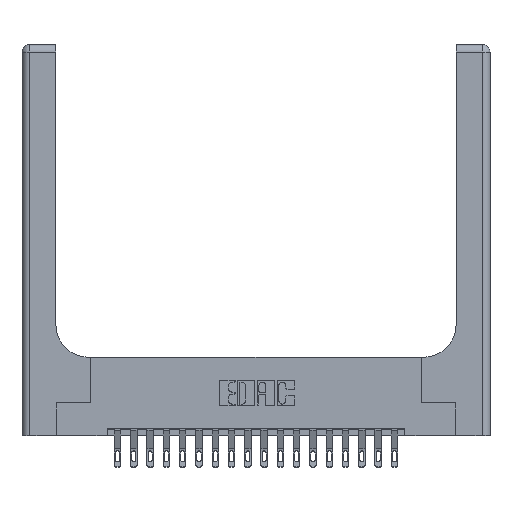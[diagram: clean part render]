
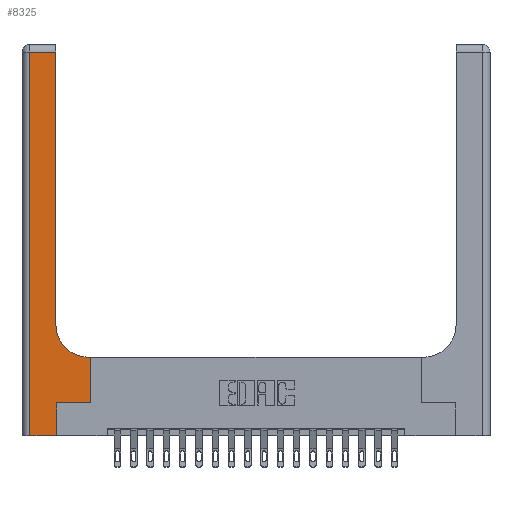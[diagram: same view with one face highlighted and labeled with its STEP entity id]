
A CAD part, top view. The second image highlights one B-rep face of the part: STEP entity #8325.
In plain terms, the highlighted planar face has unit normal (0, 0, 1).
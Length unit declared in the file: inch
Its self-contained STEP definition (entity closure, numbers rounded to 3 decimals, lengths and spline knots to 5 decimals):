
#182 = CARTESIAN_POINT ( 'NONE',  ( 0., 3., 0.37 ) ) ;
#192 = ORIENTED_EDGE ( 'NONE', *, *, #1601, .T. ) ;
#397 = PLANE ( 'NONE',  #14559 ) ;
#484 = VERTEX_POINT ( 'NONE', #10030 ) ;
#587 = LINE ( 'NONE', #1629, #3784 ) ;
#641 = FACE_OUTER_BOUND ( 'NONE', #3312, .T. ) ;
#722 = DIRECTION ( 'NONE',  ( 1., 0., 0. ) ) ;
#741 = VECTOR ( 'NONE', #9796, 39.37008 ) ;
#761 = VERTEX_POINT ( 'NONE', #2912 ) ;
#956 = LINE ( 'NONE', #8759, #11575 ) ;
#1210 = VERTEX_POINT ( 'NONE', #13691 ) ;
#1320 = LINE ( 'NONE', #3894, #5758 ) ;
#1523 = CARTESIAN_POINT ( 'NONE',  ( 0.51, 0.85, 0.37 ) ) ;
#1601 = EDGE_CURVE ( 'NONE', #15247, #5620, #1320, .T. ) ;
#1629 = CARTESIAN_POINT ( 'NONE',  ( 0.06, 3., 0.37 ) ) ;
#1920 = DIRECTION ( 'NONE',  ( 1., 0., 0. ) ) ;
#2280 = EDGE_CURVE ( 'NONE', #5620, #1210, #16123, .T. ) ;
#2809 = DIRECTION ( 'NONE',  ( 0., 1., 0. ) ) ;
#2826 = CARTESIAN_POINT ( 'NONE',  ( 0.26, 0.6, 0.37 ) ) ;
#2865 = ORIENTED_EDGE ( 'NONE', *, *, #10190, .T. ) ;
#2873 = CARTESIAN_POINT ( 'NONE',  ( 0.26, 3., 0.37 ) ) ;
#2912 = CARTESIAN_POINT ( 'NONE',  ( 0.51, 0.6, 0.37 ) ) ;
#3312 = EDGE_LOOP ( 'NONE', ( #8484, #2865, #6589, #14751, #3699, #192, #15253, #14975, #11862 ) ) ;
#3699 = ORIENTED_EDGE ( 'NONE', *, *, #14763, .T. ) ;
#3784 = VECTOR ( 'NONE', #12694, 39.37008 ) ;
#3894 = CARTESIAN_POINT ( 'NONE',  ( 0.265, 0.25, 0.37 ) ) ;
#4897 = CARTESIAN_POINT ( 'NONE',  ( 0.528, 0.25, 0.37 ) ) ;
#4983 = CARTESIAN_POINT ( 'NONE',  ( 0., 2.94, 0.37 ) ) ;
#5076 = DIRECTION ( 'NONE',  ( 0., 0., -1. ) ) ;
#5408 = CARTESIAN_POINT ( 'NONE',  ( 0.265, 0.25, 0.37 ) ) ;
#5620 = VERTEX_POINT ( 'NONE', #4897 ) ;
#5758 = VECTOR ( 'NONE', #722, 39.37008 ) ;
#6589 = ORIENTED_EDGE ( 'NONE', *, *, #9527, .T. ) ;
#6635 = EDGE_CURVE ( 'NONE', #19208, #19893, #16492, .T. ) ;
#7496 = CARTESIAN_POINT ( 'NONE',  ( 0.528, 0.25, 0.37 ) ) ;
#8325 = ADVANCED_FACE ( 'NONE', ( #641 ), #397, .F. ) ;
#8484 = ORIENTED_EDGE ( 'NONE', *, *, #6635, .T. ) ;
#8759 = CARTESIAN_POINT ( 'NONE',  ( 0.265, 0., 0.37 ) ) ;
#9527 = EDGE_CURVE ( 'NONE', #11602, #15849, #587, .T. ) ;
#9796 = DIRECTION ( 'NONE',  ( 1., 0., 0. ) ) ;
#9930 = EDGE_CURVE ( 'NONE', #1210, #761, #13692, .T. ) ;
#10030 = CARTESIAN_POINT ( 'NONE',  ( 0.265, 0., 0.37 ) ) ;
#10147 = LINE ( 'NONE', #19384, #741 ) ;
#10190 = EDGE_CURVE ( 'NONE', #19893, #11602, #10949, .T. ) ;
#10684 = DIRECTION ( 'NONE',  ( 0., 1., 0. ) ) ;
#10949 = LINE ( 'NONE', #4983, #17888 ) ;
#10997 = CARTESIAN_POINT ( 'NONE',  ( 0.26, 2.94, 0.37 ) ) ;
#11544 = DIRECTION ( 'NONE',  ( -1., 0., 0. ) ) ;
#11575 = VECTOR ( 'NONE', #13351, 39.37008 ) ;
#11602 = VERTEX_POINT ( 'NONE', #11837 ) ;
#11837 = CARTESIAN_POINT ( 'NONE',  ( 0.06, 2.94, 0.37 ) ) ;
#11862 = ORIENTED_EDGE ( 'NONE', *, *, #15612, .T. ) ;
#12471 = DIRECTION ( 'NONE',  ( -1., 0., 0. ) ) ;
#12694 = DIRECTION ( 'NONE',  ( 0., -1., 0. ) ) ;
#12967 = VECTOR ( 'NONE', #12471, 39.37008 ) ;
#13345 = CARTESIAN_POINT ( 'NONE',  ( 0.06, 0., 0.37 ) ) ;
#13351 = DIRECTION ( 'NONE',  ( 0., 1., 0. ) ) ;
#13555 = VECTOR ( 'NONE', #2809, 39.37008 ) ;
#13691 = CARTESIAN_POINT ( 'NONE',  ( 0.528, 0.6, 0.37 ) ) ;
#13692 = LINE ( 'NONE', #2826, #12967 ) ;
#13972 = CARTESIAN_POINT ( 'NONE',  ( 0.26, 0.85, 0.37 ) ) ;
#14559 = AXIS2_PLACEMENT_3D ( 'NONE', #182, #5076, #17669 ) ;
#14654 = AXIS2_PLACEMENT_3D ( 'NONE', #1523, #14708, #1920 ) ;
#14708 = DIRECTION ( 'NONE',  ( 0., 0., -1. ) ) ;
#14751 = ORIENTED_EDGE ( 'NONE', *, *, #19416, .T. ) ;
#14763 = EDGE_CURVE ( 'NONE', #484, #15247, #956, .T. ) ;
#14975 = ORIENTED_EDGE ( 'NONE', *, *, #9930, .T. ) ;
#15247 = VERTEX_POINT ( 'NONE', #5408 ) ;
#15253 = ORIENTED_EDGE ( 'NONE', *, *, #2280, .T. ) ;
#15612 = EDGE_CURVE ( 'NONE', #761, #19208, #18008, .T. ) ;
#15849 = VERTEX_POINT ( 'NONE', #13345 ) ;
#16123 = LINE ( 'NONE', #7496, #17125 ) ;
#16492 = LINE ( 'NONE', #2873, #13555 ) ;
#17125 = VECTOR ( 'NONE', #10684, 39.37008 ) ;
#17669 = DIRECTION ( 'NONE',  ( -1., 0., 0. ) ) ;
#17888 = VECTOR ( 'NONE', #11544, 39.37008 ) ;
#18008 = CIRCLE ( 'NONE', #14654, 0.25 ) ;
#19208 = VERTEX_POINT ( 'NONE', #13972 ) ;
#19384 = CARTESIAN_POINT ( 'NONE',  ( 0., 0., 0.37 ) ) ;
#19416 = EDGE_CURVE ( 'NONE', #15849, #484, #10147, .T. ) ;
#19893 = VERTEX_POINT ( 'NONE', #10997 ) ;
